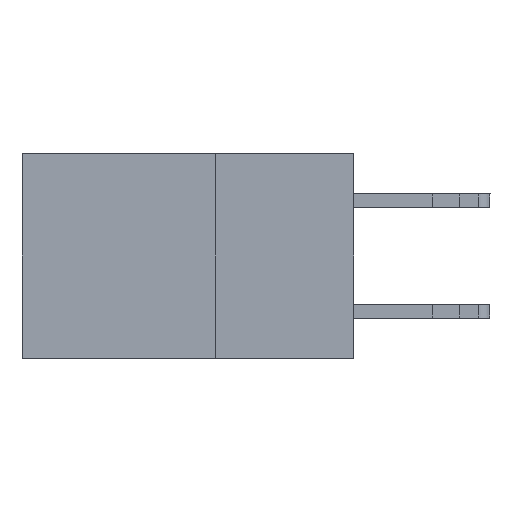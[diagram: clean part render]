
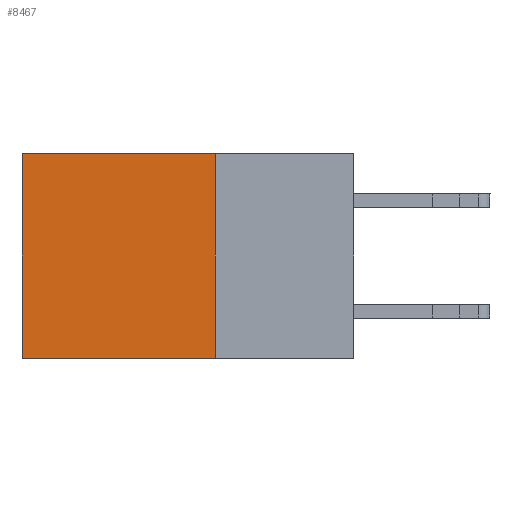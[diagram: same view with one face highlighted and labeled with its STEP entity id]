
A CAD part, left-side view. The second image highlights one B-rep face of the part: STEP entity #8467.
In plain terms, the highlighted planar face has unit normal (-1, 0, 0).
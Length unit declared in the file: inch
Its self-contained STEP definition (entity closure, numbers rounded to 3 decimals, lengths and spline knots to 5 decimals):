
#284 = CARTESIAN_POINT ( 'NONE',  ( 0.2875, 0.6, 0. ) ) ;
#1464 = CARTESIAN_POINT ( 'NONE',  ( 0.2875, 0.25, 0. ) ) ;
#2201 = EDGE_LOOP ( 'NONE', ( #15679, #16170, #12393, #18808 ) ) ;
#2320 = CARTESIAN_POINT ( 'NONE',  ( 0.2875, 0.25, -0.37 ) ) ;
#2386 = EDGE_CURVE ( 'NONE', #14079, #15864, #11470, .T. ) ;
#2502 = VECTOR ( 'NONE', #18098, 39.37008 ) ;
#3647 = PLANE ( 'NONE',  #12606 ) ;
#5605 = CARTESIAN_POINT ( 'NONE',  ( 0.2875, 0.25, 0. ) ) ;
#5634 = EDGE_CURVE ( 'NONE', #17162, #14079, #12971, .T. ) ;
#7459 = DIRECTION ( 'NONE',  ( 0., 0., -1. ) ) ;
#8467 = ADVANCED_FACE ( 'NONE', ( #12960 ), #3647, .F. ) ;
#9725 = VERTEX_POINT ( 'NONE', #18813 ) ;
#11470 = LINE ( 'NONE', #11601, #13461 ) ;
#11538 = CARTESIAN_POINT ( 'NONE',  ( 0.2875, 0.25, 0. ) ) ;
#11601 = CARTESIAN_POINT ( 'NONE',  ( 0.2875, 0.6, 0. ) ) ;
#12393 = ORIENTED_EDGE ( 'NONE', *, *, #13980, .F. ) ;
#12606 = AXIS2_PLACEMENT_3D ( 'NONE', #11538, #22745, #19905 ) ;
#12960 = FACE_OUTER_BOUND ( 'NONE', #2201, .T. ) ;
#12971 = LINE ( 'NONE', #1464, #23068 ) ;
#13461 = VECTOR ( 'NONE', #7459, 39.37008 ) ;
#13980 = EDGE_CURVE ( 'NONE', #17162, #9725, #23542, .T. ) ;
#14079 = VERTEX_POINT ( 'NONE', #284 ) ;
#14129 = CARTESIAN_POINT ( 'NONE',  ( 0.2875, 0.25, 0. ) ) ;
#14491 = EDGE_CURVE ( 'NONE', #9725, #15864, #20016, .T. ) ;
#15679 = ORIENTED_EDGE ( 'NONE', *, *, #2386, .T. ) ;
#15864 = VERTEX_POINT ( 'NONE', #21356 ) ;
#16170 = ORIENTED_EDGE ( 'NONE', *, *, #14491, .F. ) ;
#17162 = VERTEX_POINT ( 'NONE', #5605 ) ;
#18098 = DIRECTION ( 'NONE',  ( 0., 1., 0. ) ) ;
#18808 = ORIENTED_EDGE ( 'NONE', *, *, #5634, .T. ) ;
#18813 = CARTESIAN_POINT ( 'NONE',  ( 0.2875, 0.25, -0.37 ) ) ;
#19905 = DIRECTION ( 'NONE',  ( 0., 0., -1. ) ) ;
#20016 = LINE ( 'NONE', #2320, #2502 ) ;
#21356 = CARTESIAN_POINT ( 'NONE',  ( 0.2875, 0.6, -0.37 ) ) ;
#21737 = DIRECTION ( 'NONE',  ( 0., 0., -1. ) ) ;
#22745 = DIRECTION ( 'NONE',  ( 1., 0., 0. ) ) ;
#23068 = VECTOR ( 'NONE', #24709, 39.37008 ) ;
#23542 = LINE ( 'NONE', #14129, #24320 ) ;
#24320 = VECTOR ( 'NONE', #21737, 39.37008 ) ;
#24709 = DIRECTION ( 'NONE',  ( 0., 1., 0. ) ) ;
